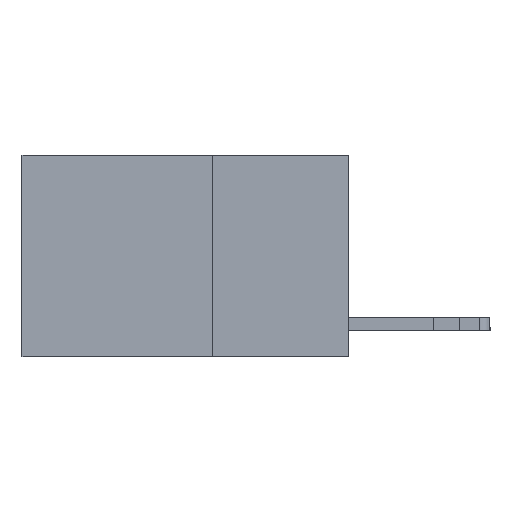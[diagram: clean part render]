
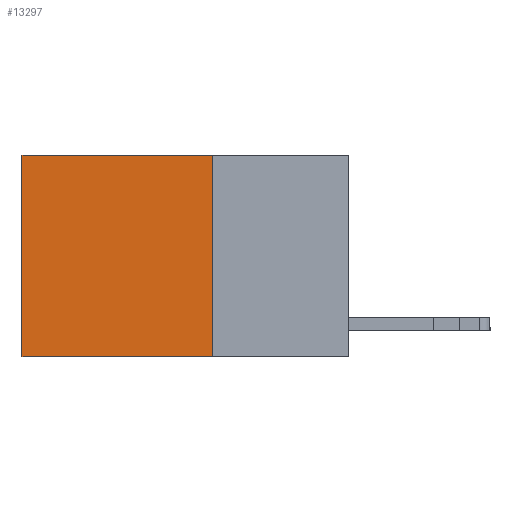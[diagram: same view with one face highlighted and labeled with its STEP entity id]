
A CAD part, left-side view. The second image highlights one B-rep face of the part: STEP entity #13297.
In plain terms, the highlighted planar face has unit normal (-1, 0, 0).
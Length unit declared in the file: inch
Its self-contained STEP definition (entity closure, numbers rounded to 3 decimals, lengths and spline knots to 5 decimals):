
#28 = VECTOR ( 'NONE', #10844, 39.37008 ) ;
#349 = VECTOR ( 'NONE', #4484, 39.37008 ) ;
#888 = CARTESIAN_POINT ( 'NONE',  ( 0.2625, 0.6, -0.37 ) ) ;
#1175 = CARTESIAN_POINT ( 'NONE',  ( 0.2625, 0.6, 0. ) ) ;
#2097 = DIRECTION ( 'NONE',  ( 1., 0., 0. ) ) ;
#2645 = LINE ( 'NONE', #14351, #12785 ) ;
#3732 = PLANE ( 'NONE',  #7838 ) ;
#3986 = DIRECTION ( 'NONE',  ( 0., 1., 0. ) ) ;
#4484 = DIRECTION ( 'NONE',  ( 0., 0., -1. ) ) ;
#4980 = CARTESIAN_POINT ( 'NONE',  ( 0.2625, 0.25, 0. ) ) ;
#5349 = EDGE_LOOP ( 'NONE', ( #12276, #8654, #13889, #15114 ) ) ;
#5703 = CARTESIAN_POINT ( 'NONE',  ( 0.2625, 0.25, 0. ) ) ;
#6525 = CARTESIAN_POINT ( 'NONE',  ( 0.2625, 0.25, -0.37 ) ) ;
#7182 = VERTEX_POINT ( 'NONE', #14722 ) ;
#7838 = AXIS2_PLACEMENT_3D ( 'NONE', #4980, #2097, #13812 ) ;
#8467 = EDGE_CURVE ( 'NONE', #7182, #14804, #10334, .T. ) ;
#8615 = CARTESIAN_POINT ( 'NONE',  ( 0.2625, 0.25, 0. ) ) ;
#8654 = ORIENTED_EDGE ( 'NONE', *, *, #18346, .F. ) ;
#10334 = LINE ( 'NONE', #8615, #349 ) ;
#10844 = DIRECTION ( 'NONE',  ( 0., 1., 0. ) ) ;
#11527 = VECTOR ( 'NONE', #3986, 39.37008 ) ;
#12276 = ORIENTED_EDGE ( 'NONE', *, *, #14503, .T. ) ;
#12287 = LINE ( 'NONE', #6525, #28 ) ;
#12325 = VERTEX_POINT ( 'NONE', #888 ) ;
#12548 = FACE_OUTER_BOUND ( 'NONE', #5349, .T. ) ;
#12785 = VECTOR ( 'NONE', #18464, 39.37008 ) ;
#13297 = ADVANCED_FACE ( 'NONE', ( #12548 ), #3732, .F. ) ;
#13754 = EDGE_CURVE ( 'NONE', #7182, #16305, #14162, .T. ) ;
#13812 = DIRECTION ( 'NONE',  ( 0., 0., -1. ) ) ;
#13889 = ORIENTED_EDGE ( 'NONE', *, *, #8467, .F. ) ;
#14162 = LINE ( 'NONE', #5703, #11527 ) ;
#14351 = CARTESIAN_POINT ( 'NONE',  ( 0.2625, 0.6, 0. ) ) ;
#14503 = EDGE_CURVE ( 'NONE', #16305, #12325, #2645, .T. ) ;
#14722 = CARTESIAN_POINT ( 'NONE',  ( 0.2625, 0.25, 0. ) ) ;
#14804 = VERTEX_POINT ( 'NONE', #16725 ) ;
#15114 = ORIENTED_EDGE ( 'NONE', *, *, #13754, .T. ) ;
#16305 = VERTEX_POINT ( 'NONE', #1175 ) ;
#16725 = CARTESIAN_POINT ( 'NONE',  ( 0.2625, 0.25, -0.37 ) ) ;
#18346 = EDGE_CURVE ( 'NONE', #14804, #12325, #12287, .T. ) ;
#18464 = DIRECTION ( 'NONE',  ( 0., 0., -1. ) ) ;
